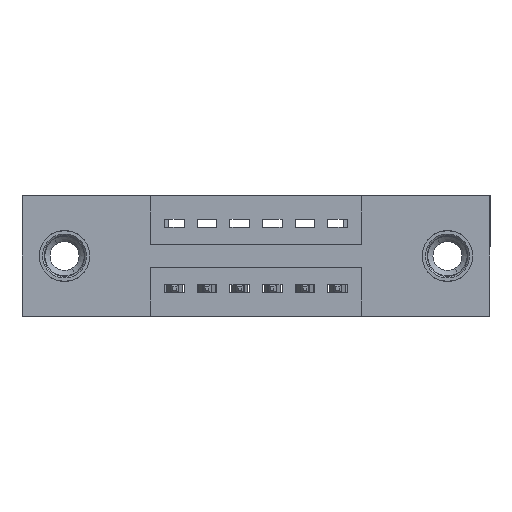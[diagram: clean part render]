
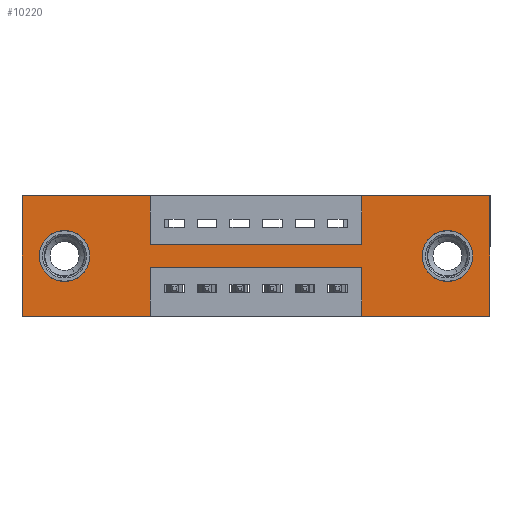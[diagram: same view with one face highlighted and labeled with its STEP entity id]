
A CAD part, front view. The second image highlights one B-rep face of the part: STEP entity #10220.
In plain terms, the highlighted planar face has unit normal (0, -1, 0).
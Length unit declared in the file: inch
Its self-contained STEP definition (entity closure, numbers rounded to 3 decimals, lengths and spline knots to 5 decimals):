
#160 = VERTEX_POINT ( 'NONE', #6826 ) ;
#292 = EDGE_CURVE ( 'NONE', #7210, #5946, #1294, .T. ) ;
#314 = CIRCLE ( 'NONE', #2799, 0.078 ) ;
#347 = DIRECTION ( 'NONE',  ( 0., 1., 0. ) ) ;
#559 = CARTESIAN_POINT ( 'NONE',  ( 1.0425, 0., -0.37 ) ) ;
#664 = LINE ( 'NONE', #11436, #7391 ) ;
#687 = LINE ( 'NONE', #4538, #3067 ) ;
#759 = FACE_OUTER_BOUND ( 'NONE', #3244, .T. ) ;
#765 = DIRECTION ( 'NONE',  ( 0., 0., 1. ) ) ;
#1132 = VERTEX_POINT ( 'NONE', #9085 ) ;
#1294 = LINE ( 'NONE', #10966, #5334 ) ;
#1299 = ORIENTED_EDGE ( 'NONE', *, *, #1774, .F. ) ;
#1332 = FACE_BOUND ( 'NONE', #4389, .T. ) ;
#1440 = DIRECTION ( 'NONE',  ( 0., 0., -1. ) ) ;
#1483 = CARTESIAN_POINT ( 'NONE',  ( 1.0425, 0., -0.37 ) ) ;
#1493 = LINE ( 'NONE', #4642, #2892 ) ;
#1656 = EDGE_CURVE ( 'NONE', #1132, #7629, #4176, .T. ) ;
#1684 = CARTESIAN_POINT ( 'NONE',  ( 0.3925, 0., -0.22 ) ) ;
#1774 = EDGE_CURVE ( 'NONE', #3445, #1976, #687, .T. ) ;
#1814 = AXIS2_PLACEMENT_3D ( 'NONE', #3205, #6853, #5786 ) ;
#1876 = VERTEX_POINT ( 'NONE', #8067 ) ;
#1958 = EDGE_CURVE ( 'NONE', #7915, #6762, #8795, .T. ) ;
#1976 = VERTEX_POINT ( 'NONE', #8567 ) ;
#2003 = DIRECTION ( 'NONE',  ( 1., 0., 0. ) ) ;
#2198 = CARTESIAN_POINT ( 'NONE',  ( 1.435, 0., 0. ) ) ;
#2345 = CARTESIAN_POINT ( 'NONE',  ( 1.305, 0., -0.263 ) ) ;
#2415 = VERTEX_POINT ( 'NONE', #2198 ) ;
#2558 = LINE ( 'NONE', #5894, #11347 ) ;
#2581 = DIRECTION ( 'NONE',  ( -1., 0., 0. ) ) ;
#2799 = AXIS2_PLACEMENT_3D ( 'NONE', #3146, #7525, #11043 ) ;
#2825 = ORIENTED_EDGE ( 'NONE', *, *, #11453, .F. ) ;
#2858 = FACE_BOUND ( 'NONE', #8466, .T. ) ;
#2887 = ORIENTED_EDGE ( 'NONE', *, *, #10380, .F. ) ;
#2892 = VECTOR ( 'NONE', #9075, 39.37008 ) ;
#2932 = CARTESIAN_POINT ( 'NONE',  ( 1.0425, 0., 0. ) ) ;
#3067 = VECTOR ( 'NONE', #5575, 39.37008 ) ;
#3146 = CARTESIAN_POINT ( 'NONE',  ( 0.13, 0., -0.185 ) ) ;
#3176 = VERTEX_POINT ( 'NONE', #5015 ) ;
#3177 = ORIENTED_EDGE ( 'NONE', *, *, #292, .F. ) ;
#3205 = CARTESIAN_POINT ( 'NONE',  ( 1.305, 0., -0.185 ) ) ;
#3244 = EDGE_LOOP ( 'NONE', ( #6496, #2887, #8718, #2825, #11047, #8838, #7589, #6958, #5144, #3177, #9883, #1299 ) ) ;
#3336 = DIRECTION ( 'NONE',  ( 0., 0., 1. ) ) ;
#3445 = VERTEX_POINT ( 'NONE', #6658 ) ;
#3594 = EDGE_CURVE ( 'NONE', #11167, #1132, #9721, .T. ) ;
#3612 = EDGE_CURVE ( 'NONE', #160, #9709, #4959, .T. ) ;
#3636 = EDGE_CURVE ( 'NONE', #7032, #3445, #9023, .T. ) ;
#3707 = VECTOR ( 'NONE', #9374, 39.37008 ) ;
#3785 = AXIS2_PLACEMENT_3D ( 'NONE', #8371, #347, #11139 ) ;
#4004 = PLANE ( 'NONE',  #5847 ) ;
#4176 = LINE ( 'NONE', #6497, #9902 ) ;
#4213 = ORIENTED_EDGE ( 'NONE', *, *, #4909, .T. ) ;
#4387 = EDGE_CURVE ( 'NONE', #1976, #7210, #2558, .T. ) ;
#4389 = EDGE_LOOP ( 'NONE', ( #5069, #4213 ) ) ;
#4455 = DIRECTION ( 'NONE',  ( 1., 0., 0. ) ) ;
#4538 = CARTESIAN_POINT ( 'NONE',  ( 0., 0., -0.37 ) ) ;
#4599 = VERTEX_POINT ( 'NONE', #5289 ) ;
#4642 = CARTESIAN_POINT ( 'NONE',  ( 1.435, 0., 0. ) ) ;
#4869 = DIRECTION ( 'NONE',  ( 0., 0., 1. ) ) ;
#4909 = EDGE_CURVE ( 'NONE', #3176, #1876, #314, .T. ) ;
#4959 = CIRCLE ( 'NONE', #1814, 0.078 ) ;
#5015 = CARTESIAN_POINT ( 'NONE',  ( 0.13, 0., -0.263 ) ) ;
#5069 = ORIENTED_EDGE ( 'NONE', *, *, #6986, .T. ) ;
#5144 = ORIENTED_EDGE ( 'NONE', *, *, #9617, .F. ) ;
#5194 = CARTESIAN_POINT ( 'NONE',  ( 0.3925, 0., -0.22 ) ) ;
#5232 = DIRECTION ( 'NONE',  ( 0., 1., 0. ) ) ;
#5289 = CARTESIAN_POINT ( 'NONE',  ( 1.435, 0., -0.37 ) ) ;
#5291 = VECTOR ( 'NONE', #9649, 39.37008 ) ;
#5334 = VECTOR ( 'NONE', #2003, 39.37008 ) ;
#5575 = DIRECTION ( 'NONE',  ( -1., 0., 0. ) ) ;
#5597 = CARTESIAN_POINT ( 'NONE',  ( 0.3925, 0., -0.15 ) ) ;
#5786 = DIRECTION ( 'NONE',  ( 0., 0., -1. ) ) ;
#5826 = DIRECTION ( 'NONE',  ( 1., 0., 0. ) ) ;
#5835 = ORIENTED_EDGE ( 'NONE', *, *, #7742, .T. ) ;
#5847 = AXIS2_PLACEMENT_3D ( 'NONE', #10257, #10178, #9328 ) ;
#5867 = CARTESIAN_POINT ( 'NONE',  ( 0.3925, 0., -0.15 ) ) ;
#5894 = CARTESIAN_POINT ( 'NONE',  ( 0., 0., 0. ) ) ;
#5946 = VERTEX_POINT ( 'NONE', #9053 ) ;
#5951 = CARTESIAN_POINT ( 'NONE',  ( 0., 0., -0.37 ) ) ;
#6098 = VECTOR ( 'NONE', #2581, 39.37008 ) ;
#6470 = ORIENTED_EDGE ( 'NONE', *, *, #3612, .T. ) ;
#6496 = ORIENTED_EDGE ( 'NONE', *, *, #3636, .F. ) ;
#6497 = CARTESIAN_POINT ( 'NONE',  ( 1.0425, 0., 0. ) ) ;
#6658 = CARTESIAN_POINT ( 'NONE',  ( 0.3925, 0., -0.37 ) ) ;
#6762 = VERTEX_POINT ( 'NONE', #7554 ) ;
#6826 = CARTESIAN_POINT ( 'NONE',  ( 1.305, 0., -0.107 ) ) ;
#6853 = DIRECTION ( 'NONE',  ( 0., 1., 0. ) ) ;
#6886 = CARTESIAN_POINT ( 'NONE',  ( 0.3925, 0., 0. ) ) ;
#6958 = ORIENTED_EDGE ( 'NONE', *, *, #3594, .F. ) ;
#6986 = EDGE_CURVE ( 'NONE', #1876, #3176, #8083, .T. ) ;
#7032 = VERTEX_POINT ( 'NONE', #1684 ) ;
#7210 = VERTEX_POINT ( 'NONE', #11001 ) ;
#7364 = VECTOR ( 'NONE', #5826, 39.37008 ) ;
#7391 = VECTOR ( 'NONE', #4455, 39.37008 ) ;
#7402 = DIRECTION ( 'NONE',  ( 0., 0., 1. ) ) ;
#7525 = DIRECTION ( 'NONE',  ( 0., 1., 0. ) ) ;
#7554 = CARTESIAN_POINT ( 'NONE',  ( 1.0425, 0., -0.22 ) ) ;
#7589 = ORIENTED_EDGE ( 'NONE', *, *, #1656, .F. ) ;
#7629 = VERTEX_POINT ( 'NONE', #2932 ) ;
#7742 = EDGE_CURVE ( 'NONE', #9709, #160, #10153, .T. ) ;
#7768 = VECTOR ( 'NONE', #1440, 39.37008 ) ;
#7915 = VERTEX_POINT ( 'NONE', #1483 ) ;
#8067 = CARTESIAN_POINT ( 'NONE',  ( 0.13, 0., -0.107 ) ) ;
#8083 = CIRCLE ( 'NONE', #10516, 0.078 ) ;
#8371 = CARTESIAN_POINT ( 'NONE',  ( 1.305, 0., -0.185 ) ) ;
#8466 = EDGE_LOOP ( 'NONE', ( #6470, #5835 ) ) ;
#8551 = EDGE_CURVE ( 'NONE', #7629, #2415, #664, .T. ) ;
#8567 = CARTESIAN_POINT ( 'NONE',  ( 0., 0., -0.37 ) ) ;
#8685 = EDGE_CURVE ( 'NONE', #2415, #4599, #1493, .T. ) ;
#8718 = ORIENTED_EDGE ( 'NONE', *, *, #1958, .F. ) ;
#8795 = LINE ( 'NONE', #559, #9213 ) ;
#8838 = ORIENTED_EDGE ( 'NONE', *, *, #8551, .F. ) ;
#8934 = LINE ( 'NONE', #5951, #5291 ) ;
#9023 = LINE ( 'NONE', #9496, #3707 ) ;
#9053 = CARTESIAN_POINT ( 'NONE',  ( 0.3925, 0., 0. ) ) ;
#9075 = DIRECTION ( 'NONE',  ( 0., 0., -1. ) ) ;
#9085 = CARTESIAN_POINT ( 'NONE',  ( 1.0425, 0., -0.15 ) ) ;
#9213 = VECTOR ( 'NONE', #4869, 39.37008 ) ;
#9328 = DIRECTION ( 'NONE',  ( 0., 0., -1. ) ) ;
#9374 = DIRECTION ( 'NONE',  ( 0., 0., -1. ) ) ;
#9496 = CARTESIAN_POINT ( 'NONE',  ( 0.3925, 0., -0.37 ) ) ;
#9588 = LINE ( 'NONE', #5194, #6098 ) ;
#9617 = EDGE_CURVE ( 'NONE', #5946, #11167, #10129, .T. ) ;
#9649 = DIRECTION ( 'NONE',  ( -1., 0., 0. ) ) ;
#9709 = VERTEX_POINT ( 'NONE', #2345 ) ;
#9721 = LINE ( 'NONE', #5867, #7364 ) ;
#9883 = ORIENTED_EDGE ( 'NONE', *, *, #4387, .F. ) ;
#9902 = VECTOR ( 'NONE', #7402, 39.37008 ) ;
#10129 = LINE ( 'NONE', #6886, #7768 ) ;
#10153 = CIRCLE ( 'NONE', #3785, 0.078 ) ;
#10178 = DIRECTION ( 'NONE',  ( 0., -1., 0. ) ) ;
#10220 = ADVANCED_FACE ( 'NONE', ( #2858, #1332, #759 ), #4004, .T. ) ;
#10257 = CARTESIAN_POINT ( 'NONE',  ( 0., 0., -0.37 ) ) ;
#10380 = EDGE_CURVE ( 'NONE', #6762, #7032, #9588, .T. ) ;
#10516 = AXIS2_PLACEMENT_3D ( 'NONE', #10588, #5232, #3336 ) ;
#10588 = CARTESIAN_POINT ( 'NONE',  ( 0.13, 0., -0.185 ) ) ;
#10966 = CARTESIAN_POINT ( 'NONE',  ( 0., 0., 0. ) ) ;
#11001 = CARTESIAN_POINT ( 'NONE',  ( 0., 0., 0. ) ) ;
#11043 = DIRECTION ( 'NONE',  ( 0., 0., 1. ) ) ;
#11047 = ORIENTED_EDGE ( 'NONE', *, *, #8685, .F. ) ;
#11139 = DIRECTION ( 'NONE',  ( 0., 0., -1. ) ) ;
#11167 = VERTEX_POINT ( 'NONE', #5597 ) ;
#11347 = VECTOR ( 'NONE', #765, 39.37008 ) ;
#11436 = CARTESIAN_POINT ( 'NONE',  ( 0., 0., 0. ) ) ;
#11453 = EDGE_CURVE ( 'NONE', #4599, #7915, #8934, .T. ) ;
